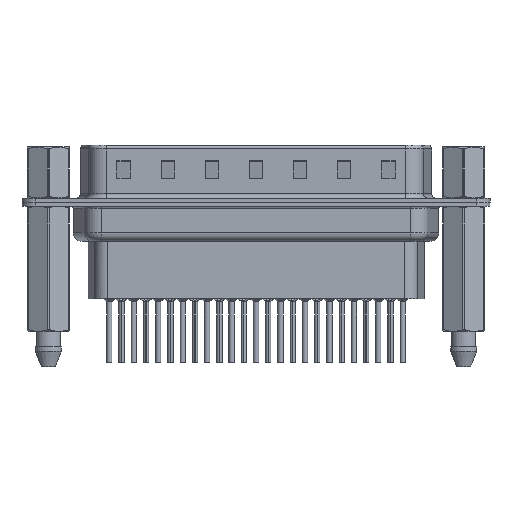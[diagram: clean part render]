
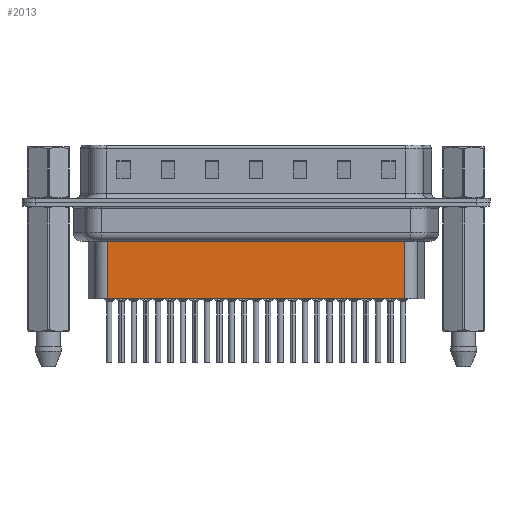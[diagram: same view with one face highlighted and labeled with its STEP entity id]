
A CAD part, front view. The second image highlights one B-rep face of the part: STEP entity #2013.
In plain terms, the highlighted planar face has unit normal (0, -1, 0).
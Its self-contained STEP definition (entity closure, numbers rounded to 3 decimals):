
#1050 = DIRECTION ( 'NONE',  ( 1., 0., 0. ) ) ;
#1482 = LINE ( 'NONE', #1649, #19370 ) ;
#1625 = CARTESIAN_POINT ( 'NONE',  ( 6.706, -3.5, -10.95 ) ) ;
#1649 = CARTESIAN_POINT ( 'NONE',  ( 6.706, -3.5, -3.1 ) ) ;
#2013 = ADVANCED_FACE ( 'NONE', ( #31418 ), #4002, .T. ) ;
#2631 = VERTEX_POINT ( 'NONE', #28659 ) ;
#2762 = LINE ( 'NONE', #7879, #32451 ) ;
#3225 = VERTEX_POINT ( 'NONE', #28724 ) ;
#4002 = PLANE ( 'NONE',  #8297 ) ;
#5532 = EDGE_CURVE ( 'NONE', #3225, #22468, #11148, .T. ) ;
#6408 = VERTEX_POINT ( 'NONE', #1625 ) ;
#6616 = CARTESIAN_POINT ( 'NONE',  ( 40.344, -3.5, -10.95 ) ) ;
#7879 = CARTESIAN_POINT ( 'NONE',  ( 6.706, -3.5, -10.95 ) ) ;
#8119 = VECTOR ( 'NONE', #20596, 1000. ) ;
#8297 = AXIS2_PLACEMENT_3D ( 'NONE', #24166, #23672, #1050 ) ;
#11148 = LINE ( 'NONE', #23717, #27411 ) ;
#12109 = ORIENTED_EDGE ( 'NONE', *, *, #14937, .F. ) ;
#14937 = EDGE_CURVE ( 'NONE', #22468, #6408, #2762, .T. ) ;
#19370 = VECTOR ( 'NONE', #32187, 1000. ) ;
#20441 = DIRECTION ( 'NONE',  ( -1., 0., 0. ) ) ;
#20596 = DIRECTION ( 'NONE',  ( -1., 0., 0. ) ) ;
#21493 = ORIENTED_EDGE ( 'NONE', *, *, #28417, .T. ) ;
#22056 = ORIENTED_EDGE ( 'NONE', *, *, #23818, .T. ) ;
#22468 = VERTEX_POINT ( 'NONE', #6616 ) ;
#23672 = DIRECTION ( 'NONE',  ( 0., -1., 0. ) ) ;
#23717 = CARTESIAN_POINT ( 'NONE',  ( 40.344, -3.5, -3.1 ) ) ;
#23818 = EDGE_CURVE ( 'NONE', #3225, #2631, #26445, .T. ) ;
#24166 = CARTESIAN_POINT ( 'NONE',  ( 6.706, -3.5, -3.1 ) ) ;
#25120 = CARTESIAN_POINT ( 'NONE',  ( 6.459, -3.5, -4.097 ) ) ;
#26355 = DIRECTION ( 'NONE',  ( 0., 0., -1. ) ) ;
#26382 = EDGE_LOOP ( 'NONE', ( #32021, #22056, #21493, #12109 ) ) ;
#26445 = LINE ( 'NONE', #25120, #8119 ) ;
#27411 = VECTOR ( 'NONE', #26355, 1000. ) ;
#28417 = EDGE_CURVE ( 'NONE', #2631, #6408, #1482, .T. ) ;
#28659 = CARTESIAN_POINT ( 'NONE',  ( 6.706, -3.5, -4.097 ) ) ;
#28724 = CARTESIAN_POINT ( 'NONE',  ( 40.344, -3.5, -4.097 ) ) ;
#31418 = FACE_OUTER_BOUND ( 'NONE', #26382, .T. ) ;
#32021 = ORIENTED_EDGE ( 'NONE', *, *, #5532, .F. ) ;
#32187 = DIRECTION ( 'NONE',  ( 0., 0., -1. ) ) ;
#32451 = VECTOR ( 'NONE', #20441, 1000. ) ;
